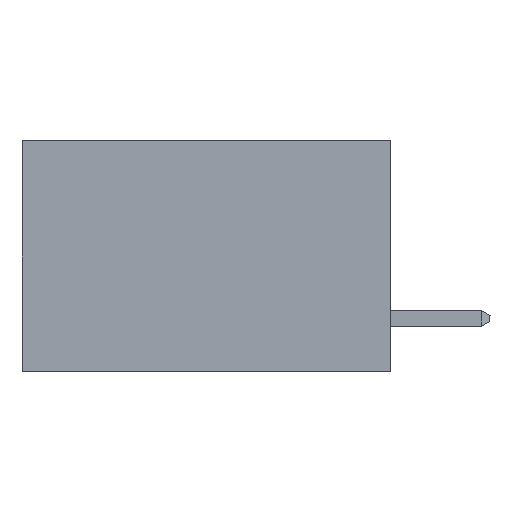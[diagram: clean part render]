
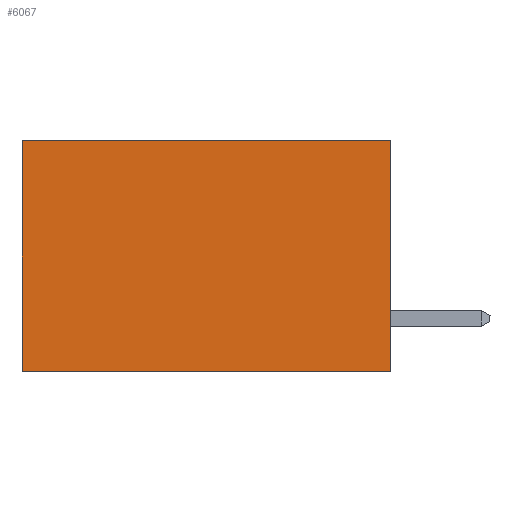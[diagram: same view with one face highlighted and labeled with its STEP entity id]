
A CAD part, left-side view. The second image highlights one B-rep face of the part: STEP entity #6067.
In plain terms, the highlighted planar face has unit normal (-1, 0, 0).
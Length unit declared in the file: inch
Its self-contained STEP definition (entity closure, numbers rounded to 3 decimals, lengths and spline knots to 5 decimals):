
#243 = CARTESIAN_POINT ( 'NONE',  ( 0.277, 0., -0.37 ) ) ;
#637 = DIRECTION ( 'NONE',  ( 0., 1., 0. ) ) ;
#720 = CARTESIAN_POINT ( 'NONE',  ( 0.277, 0., 0. ) ) ;
#832 = CARTESIAN_POINT ( 'NONE',  ( 0.277, 0., -0.37 ) ) ;
#977 = CARTESIAN_POINT ( 'NONE',  ( 0.277, 0.59, 0. ) ) ;
#1631 = FACE_OUTER_BOUND ( 'NONE', #6756, .T. ) ;
#2630 = VERTEX_POINT ( 'NONE', #977 ) ;
#2657 = EDGE_CURVE ( 'NONE', #10112, #11940, #12116, .T. ) ;
#2975 = ORIENTED_EDGE ( 'NONE', *, *, #8757, .T. ) ;
#3186 = ORIENTED_EDGE ( 'NONE', *, *, #2657, .F. ) ;
#3230 = ORIENTED_EDGE ( 'NONE', *, *, #11660, .F. ) ;
#3264 = ORIENTED_EDGE ( 'NONE', *, *, #10818, .T. ) ;
#3452 = LINE ( 'NONE', #7477, #7854 ) ;
#3976 = LINE ( 'NONE', #8968, #8689 ) ;
#4256 = CARTESIAN_POINT ( 'NONE',  ( 0.277, 0.59, -0.37 ) ) ;
#4760 = VECTOR ( 'NONE', #637, 39.37008 ) ;
#5681 = VECTOR ( 'NONE', #6176, 39.37008 ) ;
#6067 = ADVANCED_FACE ( 'NONE', ( #1631 ), #11396, .F. ) ;
#6176 = DIRECTION ( 'NONE',  ( 0., 0., -1. ) ) ;
#6614 = AXIS2_PLACEMENT_3D ( 'NONE', #11324, #11913, #11434 ) ;
#6756 = EDGE_LOOP ( 'NONE', ( #2975, #3186, #3230, #3264 ) ) ;
#7477 = CARTESIAN_POINT ( 'NONE',  ( 0.277, 0., -0.37 ) ) ;
#7854 = VECTOR ( 'NONE', #8384, 39.37008 ) ;
#8184 = LINE ( 'NONE', #4256, #5681 ) ;
#8384 = DIRECTION ( 'NONE',  ( 0., 0., -1. ) ) ;
#8689 = VECTOR ( 'NONE', #11732, 39.37008 ) ;
#8757 = EDGE_CURVE ( 'NONE', #2630, #11940, #8184, .T. ) ;
#8820 = CARTESIAN_POINT ( 'NONE',  ( 0.277, 0.59, -0.37 ) ) ;
#8968 = CARTESIAN_POINT ( 'NONE',  ( 0.277, 0., 0. ) ) ;
#10112 = VERTEX_POINT ( 'NONE', #243 ) ;
#10324 = VERTEX_POINT ( 'NONE', #720 ) ;
#10818 = EDGE_CURVE ( 'NONE', #10324, #2630, #3976, .T. ) ;
#11324 = CARTESIAN_POINT ( 'NONE',  ( 0.277, 0., -0.37 ) ) ;
#11396 = PLANE ( 'NONE',  #6614 ) ;
#11434 = DIRECTION ( 'NONE',  ( 0., 0., -1. ) ) ;
#11660 = EDGE_CURVE ( 'NONE', #10324, #10112, #3452, .T. ) ;
#11732 = DIRECTION ( 'NONE',  ( 0., 1., 0. ) ) ;
#11913 = DIRECTION ( 'NONE',  ( 1., 0., 0. ) ) ;
#11940 = VERTEX_POINT ( 'NONE', #8820 ) ;
#12116 = LINE ( 'NONE', #832, #4760 ) ;
